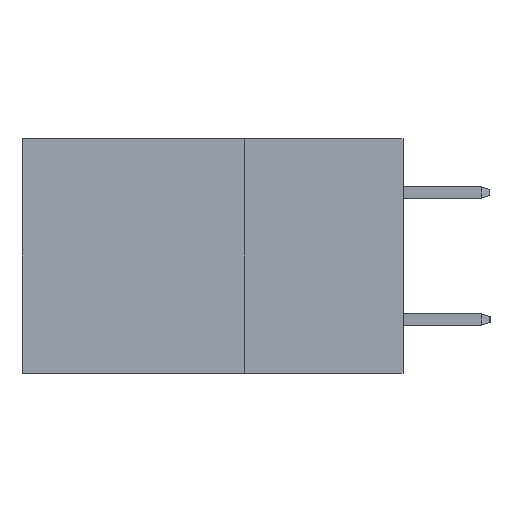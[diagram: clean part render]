
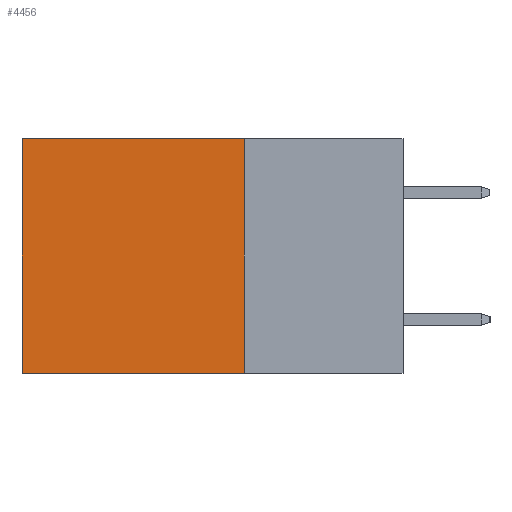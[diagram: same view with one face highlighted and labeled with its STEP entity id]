
A CAD part, left-side view. The second image highlights one B-rep face of the part: STEP entity #4456.
In plain terms, the highlighted planar face has unit normal (-1, 0, 0).
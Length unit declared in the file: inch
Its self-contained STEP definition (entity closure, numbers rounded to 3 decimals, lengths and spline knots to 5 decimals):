
#182 = EDGE_CURVE ( 'NONE', #15572, #18638, #9717, .T. ) ;
#616 = CARTESIAN_POINT ( 'NONE',  ( 0.2875, 0.6, 0. ) ) ;
#866 = EDGE_CURVE ( 'NONE', #1611, #15572, #2189, .T. ) ;
#1611 = VERTEX_POINT ( 'NONE', #4210 ) ;
#2189 = LINE ( 'NONE', #15398, #5695 ) ;
#2276 = DIRECTION ( 'NONE',  ( 0., 0., -1. ) ) ;
#2369 = PLANE ( 'NONE',  #19262 ) ;
#3559 = EDGE_LOOP ( 'NONE', ( #9003, #4681, #15419, #11263 ) ) ;
#3784 = DIRECTION ( 'NONE',  ( 1., 0., 0. ) ) ;
#3888 = CARTESIAN_POINT ( 'NONE',  ( 0.2875, 0.25, 0. ) ) ;
#4210 = CARTESIAN_POINT ( 'NONE',  ( 0.2875, 0.25, 0. ) ) ;
#4456 = ADVANCED_FACE ( 'NONE', ( #15174 ), #2369, .F. ) ;
#4681 = ORIENTED_EDGE ( 'NONE', *, *, #182, .F. ) ;
#4761 = VERTEX_POINT ( 'NONE', #5254 ) ;
#5254 = CARTESIAN_POINT ( 'NONE',  ( 0.2875, 0.6, 0. ) ) ;
#5695 = VECTOR ( 'NONE', #17231, 39.37008 ) ;
#8059 = VECTOR ( 'NONE', #14693, 39.37008 ) ;
#8557 = DIRECTION ( 'NONE',  ( 0., 0., -1. ) ) ;
#9003 = ORIENTED_EDGE ( 'NONE', *, *, #11996, .T. ) ;
#9717 = LINE ( 'NONE', #11224, #8059 ) ;
#10366 = VECTOR ( 'NONE', #16401, 39.37008 ) ;
#11105 = CARTESIAN_POINT ( 'NONE',  ( 0.2875, 0.25, 0. ) ) ;
#11224 = CARTESIAN_POINT ( 'NONE',  ( 0.2875, 0.25, -0.37 ) ) ;
#11263 = ORIENTED_EDGE ( 'NONE', *, *, #12156, .T. ) ;
#11320 = CARTESIAN_POINT ( 'NONE',  ( 0.2875, 0.6, -0.37 ) ) ;
#11996 = EDGE_CURVE ( 'NONE', #4761, #18638, #18353, .T. ) ;
#12156 = EDGE_CURVE ( 'NONE', #1611, #4761, #16076, .T. ) ;
#13462 = VECTOR ( 'NONE', #8557, 39.37008 ) ;
#14693 = DIRECTION ( 'NONE',  ( 0., 1., 0. ) ) ;
#15174 = FACE_OUTER_BOUND ( 'NONE', #3559, .T. ) ;
#15398 = CARTESIAN_POINT ( 'NONE',  ( 0.2875, 0.25, 0. ) ) ;
#15419 = ORIENTED_EDGE ( 'NONE', *, *, #866, .F. ) ;
#15572 = VERTEX_POINT ( 'NONE', #19271 ) ;
#16076 = LINE ( 'NONE', #11105, #10366 ) ;
#16401 = DIRECTION ( 'NONE',  ( 0., 1., 0. ) ) ;
#17231 = DIRECTION ( 'NONE',  ( 0., 0., -1. ) ) ;
#18353 = LINE ( 'NONE', #616, #13462 ) ;
#18638 = VERTEX_POINT ( 'NONE', #11320 ) ;
#19262 = AXIS2_PLACEMENT_3D ( 'NONE', #3888, #3784, #2276 ) ;
#19271 = CARTESIAN_POINT ( 'NONE',  ( 0.2875, 0.25, -0.37 ) ) ;
